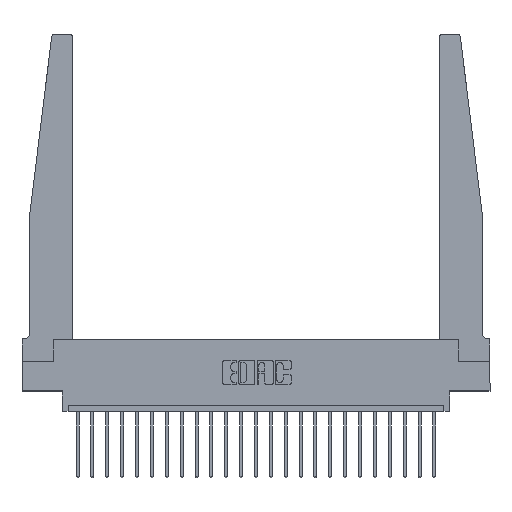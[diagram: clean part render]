
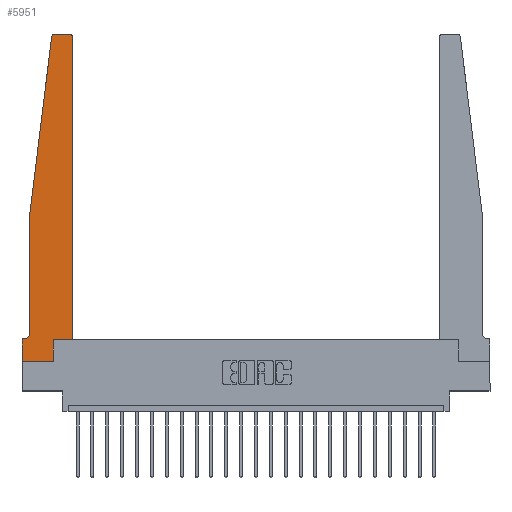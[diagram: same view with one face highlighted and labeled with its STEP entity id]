
A CAD part, top view. The second image highlights one B-rep face of the part: STEP entity #5951.
In plain terms, the highlighted planar face has unit normal (0, 0, 1).
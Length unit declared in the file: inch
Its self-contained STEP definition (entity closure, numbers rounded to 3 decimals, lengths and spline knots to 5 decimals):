
#653 = CARTESIAN_POINT ( 'NONE',  ( 0.395, 2.75, 0.37 ) ) ;
#947 = ORIENTED_EDGE ( 'NONE', *, *, #18334, .T. ) ;
#1067 = LINE ( 'NONE', #19511, #18638 ) ;
#1179 = DIRECTION ( 'NONE',  ( 1., 0., 0. ) ) ;
#1244 = DIRECTION ( 'NONE',  ( -1., 0., 0. ) ) ;
#1372 = CARTESIAN_POINT ( 'NONE',  ( 0.24675, 2.72367, 0.37 ) ) ;
#1879 = AXIS2_PLACEMENT_3D ( 'NONE', #18910, #12158, #4971 ) ;
#2058 = FACE_OUTER_BOUND ( 'NONE', #14555, .T. ) ;
#2089 = VECTOR ( 'NONE', #1179, 39.37008 ) ;
#2148 = VERTEX_POINT ( 'NONE', #16411 ) ;
#2407 = DIRECTION ( 'NONE',  ( 1., 0., 0. ) ) ;
#2464 = VECTOR ( 'NONE', #15445, 39.37008 ) ;
#2492 = CARTESIAN_POINT ( 'NONE',  ( 0., 0., 0.37 ) ) ;
#3509 = AXIS2_PLACEMENT_3D ( 'NONE', #8485, #20807, #7665 ) ;
#3643 = VERTEX_POINT ( 'NONE', #8652 ) ;
#3816 = VERTEX_POINT ( 'NONE', #16209 ) ;
#4134 = LINE ( 'NONE', #9492, #19255 ) ;
#4636 = CARTESIAN_POINT ( 'NONE',  ( 0., 0., 0.37 ) ) ;
#4679 = VECTOR ( 'NONE', #21255, 39.37008 ) ;
#4828 = CARTESIAN_POINT ( 'NONE',  ( 0., 0., 0.37 ) ) ;
#4971 = DIRECTION ( 'NONE',  ( 1., 0., 0. ) ) ;
#5508 = DIRECTION ( 'NONE',  ( 0., 1., 0. ) ) ;
#5606 = PLANE ( 'NONE',  #14612 ) ;
#5951 = ADVANCED_FACE ( 'NONE', ( #2058 ), #5606, .T. ) ;
#6657 = CARTESIAN_POINT ( 'NONE',  ( 0.065, 0.2375, 0.37 ) ) ;
#6704 = DIRECTION ( 'NONE',  ( 0., 0., -1. ) ) ;
#7665 = DIRECTION ( 'NONE',  ( 1., 0., 0. ) ) ;
#7789 = EDGE_CURVE ( 'NONE', #9583, #7940, #9404, .T. ) ;
#7856 = EDGE_CURVE ( 'NONE', #21802, #3816, #19271, .T. ) ;
#7940 = VERTEX_POINT ( 'NONE', #13136 ) ;
#8030 = ORIENTED_EDGE ( 'NONE', *, *, #10512, .T. ) ;
#8288 = AXIS2_PLACEMENT_3D ( 'NONE', #13869, #6704, #8464 ) ;
#8343 = EDGE_CURVE ( 'NONE', #7940, #3643, #14858, .T. ) ;
#8464 = DIRECTION ( 'NONE',  ( -1., 0., 0. ) ) ;
#8485 = CARTESIAN_POINT ( 'NONE',  ( 0.27653, 2.72, 0.37 ) ) ;
#8652 = CARTESIAN_POINT ( 'NONE',  ( 0., 0.1875, 0.37 ) ) ;
#9024 = CARTESIAN_POINT ( 'NONE',  ( 0.065, 0.1875, 0.37 ) ) ;
#9404 = CIRCLE ( 'NONE', #8288, 0.05 ) ;
#9492 = CARTESIAN_POINT ( 'NONE',  ( 0.425, 0.18, 0.37 ) ) ;
#9583 = VERTEX_POINT ( 'NONE', #6657 ) ;
#10091 = EDGE_CURVE ( 'NONE', #18316, #2148, #20281, .T. ) ;
#10512 = EDGE_CURVE ( 'NONE', #20733, #12906, #1067, .T. ) ;
#10718 = DIRECTION ( 'NONE',  ( -1., 0., 0. ) ) ;
#10799 = CARTESIAN_POINT ( 'NONE',  ( 0.065, 1.25, 0.37 ) ) ;
#11188 = CARTESIAN_POINT ( 'NONE',  ( 0.25, 2.75, 0.37 ) ) ;
#11235 = VECTOR ( 'NONE', #22374, 39.37008 ) ;
#11591 = EDGE_CURVE ( 'NONE', #2148, #21802, #17205, .T. ) ;
#12030 = ORIENTED_EDGE ( 'NONE', *, *, #10091, .T. ) ;
#12073 = ORIENTED_EDGE ( 'NONE', *, *, #16627, .T. ) ;
#12128 = LINE ( 'NONE', #4828, #2464 ) ;
#12158 = DIRECTION ( 'NONE',  ( 0., 0., 1. ) ) ;
#12368 = VERTEX_POINT ( 'NONE', #4636 ) ;
#12383 = CARTESIAN_POINT ( 'NONE',  ( 0.425, 2.72, 0.37 ) ) ;
#12906 = VERTEX_POINT ( 'NONE', #17511 ) ;
#13136 = CARTESIAN_POINT ( 'NONE',  ( 0.015, 0.1875, 0.37 ) ) ;
#13231 = DIRECTION ( 'NONE',  ( 0., 1., 0. ) ) ;
#13332 = ORIENTED_EDGE ( 'NONE', *, *, #7856, .T. ) ;
#13633 = EDGE_CURVE ( 'NONE', #3643, #12368, #17669, .T. ) ;
#13869 = CARTESIAN_POINT ( 'NONE',  ( 0.015, 0.2375, 0.37 ) ) ;
#14003 = ORIENTED_EDGE ( 'NONE', *, *, #15735, .T. ) ;
#14152 = ORIENTED_EDGE ( 'NONE', *, *, #11591, .T. ) ;
#14555 = EDGE_LOOP ( 'NONE', ( #12030, #14152, #13332, #12073, #21040, #22745, #19716, #14003, #8030, #947, #16831, #21228 ) ) ;
#14612 = AXIS2_PLACEMENT_3D ( 'NONE', #19907, #18174, #2407 ) ;
#14858 = LINE ( 'NONE', #9024, #20078 ) ;
#14982 = CARTESIAN_POINT ( 'NONE',  ( 0.2605, 0., 0.37 ) ) ;
#15068 = VERTEX_POINT ( 'NONE', #18358 ) ;
#15311 = CARTESIAN_POINT ( 'NONE',  ( 0.065, 1.25, 0.37 ) ) ;
#15445 = DIRECTION ( 'NONE',  ( 1., 0., 0. ) ) ;
#15735 = EDGE_CURVE ( 'NONE', #12368, #20733, #12128, .T. ) ;
#16209 = CARTESIAN_POINT ( 'NONE',  ( 0.065, 1.25, 0.37 ) ) ;
#16411 = CARTESIAN_POINT ( 'NONE',  ( 0.27653, 2.75, 0.37 ) ) ;
#16549 = CIRCLE ( 'NONE', #1879, 0.03 ) ;
#16571 = DIRECTION ( 'NONE',  ( 0., -1., 0. ) ) ;
#16627 = EDGE_CURVE ( 'NONE', #3816, #9583, #21678, .T. ) ;
#16831 = ORIENTED_EDGE ( 'NONE', *, *, #21695, .T. ) ;
#17058 = CARTESIAN_POINT ( 'NONE',  ( 0.425, 0.18, 0.37 ) ) ;
#17205 = CIRCLE ( 'NONE', #3509, 0.03 ) ;
#17511 = CARTESIAN_POINT ( 'NONE',  ( 0.2605, 0.18, 0.37 ) ) ;
#17669 = LINE ( 'NONE', #2492, #20410 ) ;
#18174 = DIRECTION ( 'NONE',  ( 0., 0., 1. ) ) ;
#18316 = VERTEX_POINT ( 'NONE', #653 ) ;
#18334 = EDGE_CURVE ( 'NONE', #12906, #15068, #20496, .T. ) ;
#18358 = CARTESIAN_POINT ( 'NONE',  ( 0.425, 0.18, 0.37 ) ) ;
#18638 = VECTOR ( 'NONE', #5508, 39.37008 ) ;
#18659 = VECTOR ( 'NONE', #1244, 39.37008 ) ;
#18910 = CARTESIAN_POINT ( 'NONE',  ( 0.395, 2.72, 0.37 ) ) ;
#18958 = VERTEX_POINT ( 'NONE', #12383 ) ;
#19255 = VECTOR ( 'NONE', #13231, 39.37008 ) ;
#19271 = LINE ( 'NONE', #10799, #4679 ) ;
#19511 = CARTESIAN_POINT ( 'NONE',  ( 0.2605, 0.18, 0.37 ) ) ;
#19716 = ORIENTED_EDGE ( 'NONE', *, *, #13633, .T. ) ;
#19907 = CARTESIAN_POINT ( 'NONE',  ( 0., 0.1875, 0.37 ) ) ;
#20078 = VECTOR ( 'NONE', #10718, 39.37008 ) ;
#20281 = LINE ( 'NONE', #11188, #18659 ) ;
#20410 = VECTOR ( 'NONE', #16571, 39.37008 ) ;
#20496 = LINE ( 'NONE', #17058, #2089 ) ;
#20733 = VERTEX_POINT ( 'NONE', #14982 ) ;
#20760 = EDGE_CURVE ( 'NONE', #18958, #18316, #16549, .T. ) ;
#20807 = DIRECTION ( 'NONE',  ( 0., 0., 1. ) ) ;
#21040 = ORIENTED_EDGE ( 'NONE', *, *, #7789, .T. ) ;
#21228 = ORIENTED_EDGE ( 'NONE', *, *, #20760, .T. ) ;
#21255 = DIRECTION ( 'NONE',  ( -0.122, -0.992, 0. ) ) ;
#21678 = LINE ( 'NONE', #15311, #11235 ) ;
#21695 = EDGE_CURVE ( 'NONE', #15068, #18958, #4134, .T. ) ;
#21802 = VERTEX_POINT ( 'NONE', #1372 ) ;
#22374 = DIRECTION ( 'NONE',  ( 0., -1., 0. ) ) ;
#22745 = ORIENTED_EDGE ( 'NONE', *, *, #8343, .T. ) ;
